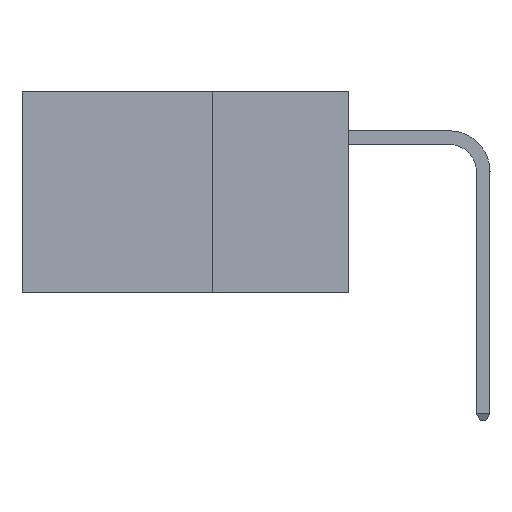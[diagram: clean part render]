
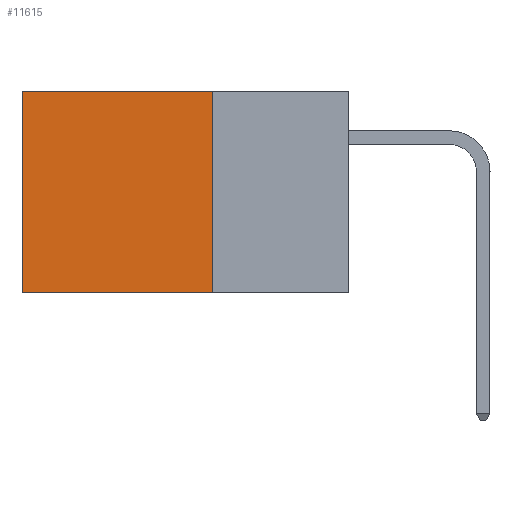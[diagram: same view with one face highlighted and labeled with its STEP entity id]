
A CAD part, left-side view. The second image highlights one B-rep face of the part: STEP entity #11615.
In plain terms, the highlighted planar face has unit normal (-1, 0, 0).
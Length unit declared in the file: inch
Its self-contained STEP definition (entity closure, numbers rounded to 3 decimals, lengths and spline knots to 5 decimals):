
#422 = VECTOR ( 'NONE', #3523, 39.37008 ) ;
#467 = CARTESIAN_POINT ( 'NONE',  ( 0.2875, 0.25, 0. ) ) ;
#943 = CARTESIAN_POINT ( 'NONE',  ( 0.2875, 0.25, 0. ) ) ;
#3009 = VECTOR ( 'NONE', #10338, 39.37008 ) ;
#3523 = DIRECTION ( 'NONE',  ( 0., 1., 0. ) ) ;
#3792 = EDGE_CURVE ( 'NONE', #9895, #9310, #8762, .T. ) ;
#3912 = EDGE_CURVE ( 'NONE', #9310, #12440, #13236, .T. ) ;
#4041 = LINE ( 'NONE', #17661, #12918 ) ;
#4066 = EDGE_CURVE ( 'NONE', #17173, #12440, #17856, .T. ) ;
#5408 = DIRECTION ( 'NONE',  ( 0., 0., -1. ) ) ;
#5668 = EDGE_CURVE ( 'NONE', #9895, #17173, #4041, .T. ) ;
#5839 = CARTESIAN_POINT ( 'NONE',  ( 0.2875, 0.25, 0. ) ) ;
#6734 = DIRECTION ( 'NONE',  ( 0., 1., 0. ) ) ;
#7702 = ORIENTED_EDGE ( 'NONE', *, *, #4066, .T. ) ;
#7984 = DIRECTION ( 'NONE',  ( 1., 0., 0. ) ) ;
#8581 = ORIENTED_EDGE ( 'NONE', *, *, #3912, .F. ) ;
#8762 = LINE ( 'NONE', #467, #3009 ) ;
#9271 = PLANE ( 'NONE',  #17572 ) ;
#9310 = VERTEX_POINT ( 'NONE', #12609 ) ;
#9420 = EDGE_LOOP ( 'NONE', ( #7702, #8581, #11307, #11571 ) ) ;
#9895 = VERTEX_POINT ( 'NONE', #5839 ) ;
#10338 = DIRECTION ( 'NONE',  ( 0., 0., -1. ) ) ;
#10598 = CARTESIAN_POINT ( 'NONE',  ( 0.2875, 0.6, -0.37 ) ) ;
#11307 = ORIENTED_EDGE ( 'NONE', *, *, #3792, .F. ) ;
#11571 = ORIENTED_EDGE ( 'NONE', *, *, #5668, .T. ) ;
#11615 = ADVANCED_FACE ( 'NONE', ( #16346 ), #9271, .F. ) ;
#11793 = CARTESIAN_POINT ( 'NONE',  ( 0.2875, 0.25, -0.37 ) ) ;
#12369 = CARTESIAN_POINT ( 'NONE',  ( 0.2875, 0.6, 0. ) ) ;
#12440 = VERTEX_POINT ( 'NONE', #10598 ) ;
#12609 = CARTESIAN_POINT ( 'NONE',  ( 0.2875, 0.25, -0.37 ) ) ;
#12918 = VECTOR ( 'NONE', #6734, 39.37008 ) ;
#13236 = LINE ( 'NONE', #11793, #422 ) ;
#14975 = DIRECTION ( 'NONE',  ( 0., 0., -1. ) ) ;
#16346 = FACE_OUTER_BOUND ( 'NONE', #9420, .T. ) ;
#16352 = VECTOR ( 'NONE', #5408, 39.37008 ) ;
#16405 = CARTESIAN_POINT ( 'NONE',  ( 0.2875, 0.6, 0. ) ) ;
#17173 = VERTEX_POINT ( 'NONE', #12369 ) ;
#17572 = AXIS2_PLACEMENT_3D ( 'NONE', #943, #7984, #14975 ) ;
#17661 = CARTESIAN_POINT ( 'NONE',  ( 0.2875, 0.25, 0. ) ) ;
#17856 = LINE ( 'NONE', #16405, #16352 ) ;
